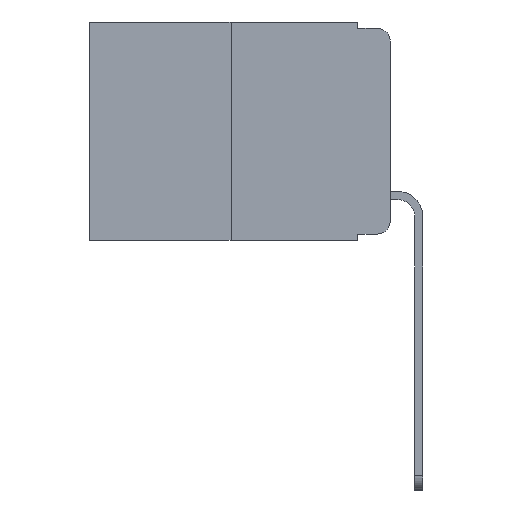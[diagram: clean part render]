
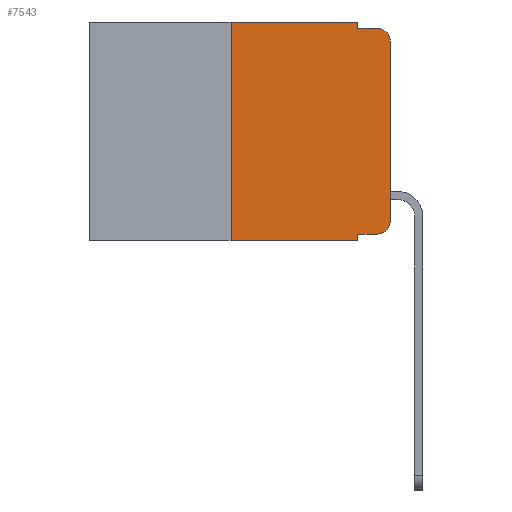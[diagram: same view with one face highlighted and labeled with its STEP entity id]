
A CAD part, left-side view. The second image highlights one B-rep face of the part: STEP entity #7543.
In plain terms, the highlighted planar face has unit normal (-1, 0, 0).
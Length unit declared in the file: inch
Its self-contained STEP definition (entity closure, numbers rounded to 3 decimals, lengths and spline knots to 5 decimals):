
#342 = EDGE_CURVE ( 'NONE', #10532, #5882, #9646, .T. ) ;
#742 = DIRECTION ( 'NONE',  ( 0., 0., -1. ) ) ;
#900 = VECTOR ( 'NONE', #11336, 39.37008 ) ;
#1092 = ORIENTED_EDGE ( 'NONE', *, *, #1723, .T. ) ;
#1267 = VECTOR ( 'NONE', #4632, 39.37008 ) ;
#1311 = VERTEX_POINT ( 'NONE', #11543 ) ;
#1407 = AXIS2_PLACEMENT_3D ( 'NONE', #3572, #2367, #5235 ) ;
#1410 = VERTEX_POINT ( 'NONE', #9189 ) ;
#1643 = LINE ( 'NONE', #2767, #1267 ) ;
#1723 = EDGE_CURVE ( 'NONE', #11054, #9119, #8529, .T. ) ;
#2103 = DIRECTION ( 'NONE',  ( 0., -1., 0. ) ) ;
#2107 = CARTESIAN_POINT ( 'NONE',  ( 0., 0.02, -0.313 ) ) ;
#2207 = FACE_OUTER_BOUND ( 'NONE', #2308, .T. ) ;
#2308 = EDGE_LOOP ( 'NONE', ( #5939, #8504, #9063, #11714, #10166, #8380, #1092, #5101, #5405, #12362 ) ) ;
#2327 = LINE ( 'NONE', #4498, #9901 ) ;
#2328 = EDGE_CURVE ( 'NONE', #7089, #3099, #8092, .T. ) ;
#2329 = EDGE_CURVE ( 'NONE', #3099, #6952, #5818, .T. ) ;
#2367 = DIRECTION ( 'NONE',  ( -1., 0., 0. ) ) ;
#2370 = EDGE_CURVE ( 'NONE', #1410, #6952, #7574, .T. ) ;
#2391 = EDGE_CURVE ( 'NONE', #5882, #1410, #2327, .T. ) ;
#2419 = EDGE_CURVE ( 'NONE', #11054, #10532, #4963, .T. ) ;
#2431 = EDGE_CURVE ( 'NONE', #1311, #9119, #1643, .T. ) ;
#2436 = EDGE_CURVE ( 'NONE', #1311, #9263, #8788, .T. ) ;
#2457 = EDGE_CURVE ( 'NONE', #9263, #7089, #3580, .T. ) ;
#2555 = DIRECTION ( 'NONE',  ( 0., 0., -1. ) ) ;
#2767 = CARTESIAN_POINT ( 'NONE',  ( 0., 0.051, 0. ) ) ;
#3099 = VERTEX_POINT ( 'NONE', #10252 ) ;
#3311 = CARTESIAN_POINT ( 'NONE',  ( 0., 0., -0.313 ) ) ;
#3521 = CARTESIAN_POINT ( 'NONE',  ( 0., 0., 0. ) ) ;
#3572 = CARTESIAN_POINT ( 'NONE',  ( 0., 0.02, -0.03 ) ) ;
#3580 = CIRCLE ( 'NONE', #6724, 0.02 ) ;
#4498 = CARTESIAN_POINT ( 'NONE',  ( 0., 0.051, 0. ) ) ;
#4632 = DIRECTION ( 'NONE',  ( 0., 0., -1. ) ) ;
#4963 = LINE ( 'NONE', #9505, #9335 ) ;
#5101 = ORIENTED_EDGE ( 'NONE', *, *, #2431, .F. ) ;
#5235 = DIRECTION ( 'NONE',  ( 0., 0., -1. ) ) ;
#5256 = VECTOR ( 'NONE', #5990, 39.37008 ) ;
#5334 = DIRECTION ( 'NONE',  ( 0., 0., 1. ) ) ;
#5405 = ORIENTED_EDGE ( 'NONE', *, *, #2436, .T. ) ;
#5818 = CIRCLE ( 'NONE', #1407, 0.02 ) ;
#5882 = VERTEX_POINT ( 'NONE', #11980 ) ;
#5939 = ORIENTED_EDGE ( 'NONE', *, *, #2328, .T. ) ;
#5990 = DIRECTION ( 'NONE',  ( 0., -1., 0. ) ) ;
#6030 = CARTESIAN_POINT ( 'NONE',  ( 0., 0.051, -0.01 ) ) ;
#6249 = VECTOR ( 'NONE', #10225, 39.37008 ) ;
#6588 = CARTESIAN_POINT ( 'NONE',  ( 0., 0.473, -0.343 ) ) ;
#6593 = PLANE ( 'NONE',  #10998 ) ;
#6724 = AXIS2_PLACEMENT_3D ( 'NONE', #2107, #9097, #742 ) ;
#6786 = DIRECTION ( 'NONE',  ( 0., 0., -1. ) ) ;
#6952 = VERTEX_POINT ( 'NONE', #7991 ) ;
#7089 = VERTEX_POINT ( 'NONE', #3311 ) ;
#7452 = CARTESIAN_POINT ( 'NONE',  ( 0., 0.051, -0.333 ) ) ;
#7543 = ADVANCED_FACE ( 'NONE', ( #2207 ), #6593, .F. ) ;
#7574 = LINE ( 'NONE', #6030, #5256 ) ;
#7991 = CARTESIAN_POINT ( 'NONE',  ( 0., 0.02, -0.01 ) ) ;
#8092 = LINE ( 'NONE', #3521, #10764 ) ;
#8275 = CARTESIAN_POINT ( 'NONE',  ( 0., 0.473, 0. ) ) ;
#8320 = DIRECTION ( 'NONE',  ( 1., 0., 0. ) ) ;
#8380 = ORIENTED_EDGE ( 'NONE', *, *, #2419, .F. ) ;
#8504 = ORIENTED_EDGE ( 'NONE', *, *, #2329, .T. ) ;
#8529 = LINE ( 'NONE', #6588, #6249 ) ;
#8788 = LINE ( 'NONE', #7452, #900 ) ;
#9063 = ORIENTED_EDGE ( 'NONE', *, *, #2370, .F. ) ;
#9097 = DIRECTION ( 'NONE',  ( -1., 0., 0. ) ) ;
#9119 = VERTEX_POINT ( 'NONE', #10183 ) ;
#9189 = CARTESIAN_POINT ( 'NONE',  ( 0., 0.051, -0.01 ) ) ;
#9263 = VERTEX_POINT ( 'NONE', #9439 ) ;
#9335 = VECTOR ( 'NONE', #10250, 39.37008 ) ;
#9439 = CARTESIAN_POINT ( 'NONE',  ( 0., 0.02, -0.333 ) ) ;
#9505 = CARTESIAN_POINT ( 'NONE',  ( 0., 0.25, 0. ) ) ;
#9646 = LINE ( 'NONE', #12069, #11488 ) ;
#9777 = CARTESIAN_POINT ( 'NONE',  ( 0., 0.25, 0. ) ) ;
#9901 = VECTOR ( 'NONE', #6786, 39.37008 ) ;
#10166 = ORIENTED_EDGE ( 'NONE', *, *, #342, .F. ) ;
#10183 = CARTESIAN_POINT ( 'NONE',  ( 0., 0.051, -0.343 ) ) ;
#10225 = DIRECTION ( 'NONE',  ( 0., -1., 0. ) ) ;
#10250 = DIRECTION ( 'NONE',  ( 0., 0., 1. ) ) ;
#10252 = CARTESIAN_POINT ( 'NONE',  ( 0., 0., -0.03 ) ) ;
#10532 = VERTEX_POINT ( 'NONE', #9777 ) ;
#10764 = VECTOR ( 'NONE', #5334, 39.37008 ) ;
#10998 = AXIS2_PLACEMENT_3D ( 'NONE', #8275, #8320, #2555 ) ;
#11054 = VERTEX_POINT ( 'NONE', #11978 ) ;
#11336 = DIRECTION ( 'NONE',  ( 0., -1., 0. ) ) ;
#11488 = VECTOR ( 'NONE', #2103, 39.37008 ) ;
#11543 = CARTESIAN_POINT ( 'NONE',  ( 0., 0.051, -0.333 ) ) ;
#11714 = ORIENTED_EDGE ( 'NONE', *, *, #2391, .F. ) ;
#11978 = CARTESIAN_POINT ( 'NONE',  ( 0., 0.25, -0.343 ) ) ;
#11980 = CARTESIAN_POINT ( 'NONE',  ( 0., 0.051, 0. ) ) ;
#12069 = CARTESIAN_POINT ( 'NONE',  ( 0., 0.473, 0. ) ) ;
#12362 = ORIENTED_EDGE ( 'NONE', *, *, #2457, .T. ) ;
